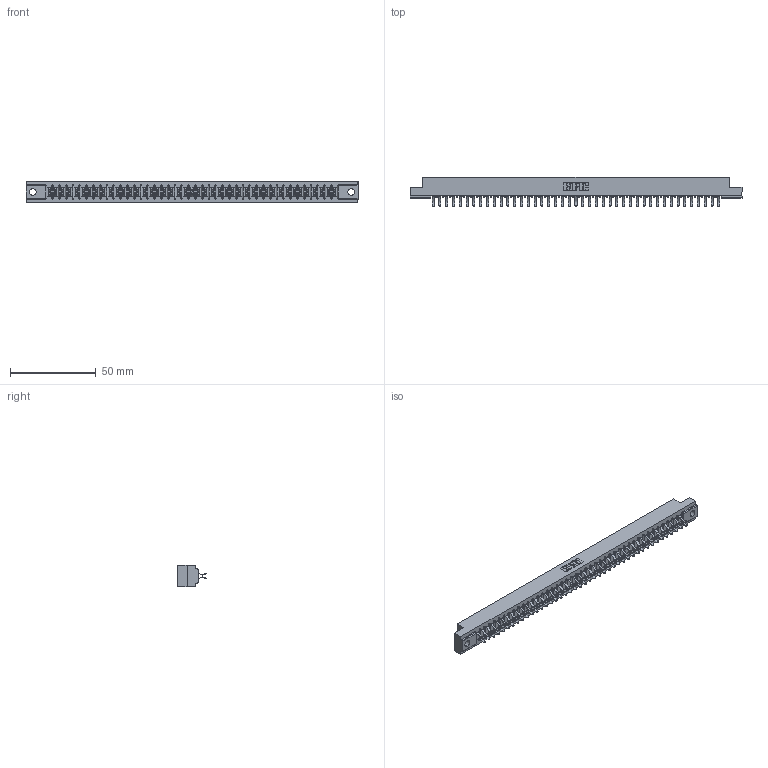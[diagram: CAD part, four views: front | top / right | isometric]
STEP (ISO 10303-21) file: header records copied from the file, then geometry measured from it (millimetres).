
FILE_DESCRIPTION (( 'STEP AP203' ), '1' );
FILE_NAME ('807-086-556-202.STEP', '2021-07-20T20:07:16', ( '' ), ( '' ), 'SwSTEP 2.0', 'SolidWorks 2020', '' );
FILE_SCHEMA (( 'CONFIG_CONTROL_DESIGN' ));
Length unit declared in the file: inch
Products named in the file (3): 807 Part_.128 Dia Mounting Holes; 307-290-001_556; 807-086-556-202
Assembly tree (87 placements, depth 2):
  807-086-556-202
    807 Part_.128 Dia Mounting Holes
    307-290-001_556  x86
Bounding box: 193.4 x 16.97 x 12.7 mm (x, y, z)
Volume: 20469 mm3; surface area: 24640.2 mm2
Topology: 87 solids, 87 shells, 4462 faces, 12535 edges, 8122 vertices
Faces by surface type: plane 2908, cylinder 1466, sphere 88
Entity records: 38222 total; most frequent: CARTESIAN_POINT 6251, ORIENTED_EDGE 6194, DIRECTION 6123, EDGE_CURVE 3097, LINE 2375, VECTOR 2375, VERTEX_POINT 2002, AXIS2_PLACEMENT_3D 1874
